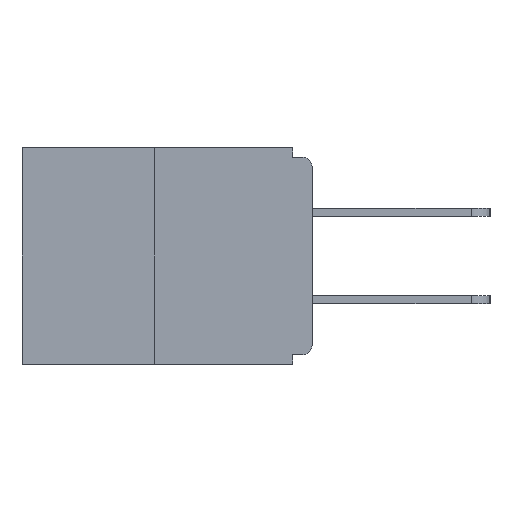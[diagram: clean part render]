
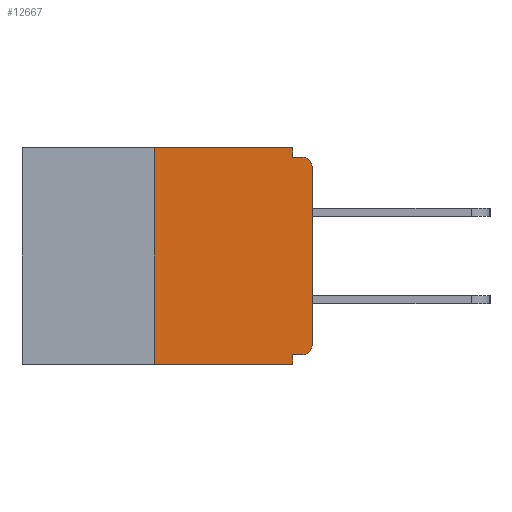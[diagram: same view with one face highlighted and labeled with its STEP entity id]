
A CAD part, left-side view. The second image highlights one B-rep face of the part: STEP entity #12667.
In plain terms, the highlighted planar face has unit normal (-1, 0, 0).
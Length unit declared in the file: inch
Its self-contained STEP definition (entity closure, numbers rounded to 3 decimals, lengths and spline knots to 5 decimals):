
#383 = CARTESIAN_POINT ( 'NONE',  ( 0., 0.25, 0. ) ) ;
#677 = CARTESIAN_POINT ( 'NONE',  ( 0., 0.015, -0.328 ) ) ;
#772 = VERTEX_POINT ( 'NONE', #23433 ) ;
#1003 = LINE ( 'NONE', #21368, #7457 ) ;
#1056 = VECTOR ( 'NONE', #14435, 39.37008 ) ;
#1057 = ORIENTED_EDGE ( 'NONE', *, *, #9455, .F. ) ;
#1495 = CARTESIAN_POINT ( 'NONE',  ( 0., 0., -0.03 ) ) ;
#1531 = DIRECTION ( 'NONE',  ( 0., 0., -1. ) ) ;
#1611 = FACE_OUTER_BOUND ( 'NONE', #10040, .T. ) ;
#2219 = EDGE_CURVE ( 'NONE', #25067, #6807, #1003, .T. ) ;
#2502 = CARTESIAN_POINT ( 'NONE',  ( 0., 0.031, 0. ) ) ;
#2650 = AXIS2_PLACEMENT_3D ( 'NONE', #13484, #15446, #21336 ) ;
#2707 = VERTEX_POINT ( 'NONE', #383 ) ;
#2754 = LINE ( 'NONE', #25011, #20819 ) ;
#3315 = VECTOR ( 'NONE', #22882, 39.37008 ) ;
#3384 = VECTOR ( 'NONE', #14317, 39.37008 ) ;
#3428 = DIRECTION ( 'NONE',  ( 0., 0., 1. ) ) ;
#3651 = ORIENTED_EDGE ( 'NONE', *, *, #4629, .T. ) ;
#3941 = CARTESIAN_POINT ( 'NONE',  ( 0., 0., -0.313 ) ) ;
#4145 = DIRECTION ( 'NONE',  ( 1., 0., 0. ) ) ;
#4515 = EDGE_CURVE ( 'NONE', #20510, #12137, #5167, .T. ) ;
#4629 = EDGE_CURVE ( 'NONE', #15922, #23898, #8237, .T. ) ;
#4657 = EDGE_CURVE ( 'NONE', #17514, #12137, #18951, .T. ) ;
#4662 = CARTESIAN_POINT ( 'NONE',  ( 0., 0.015, -0.03 ) ) ;
#5167 = LINE ( 'NONE', #20684, #3315 ) ;
#5619 = EDGE_CURVE ( 'NONE', #15922, #25067, #13058, .T. ) ;
#6807 = VERTEX_POINT ( 'NONE', #19001 ) ;
#6842 = CARTESIAN_POINT ( 'NONE',  ( 0., 0., -0.328 ) ) ;
#7069 = AXIS2_PLACEMENT_3D ( 'NONE', #10222, #4145, #17853 ) ;
#7457 = VECTOR ( 'NONE', #1531, 39.37008 ) ;
#8237 = CIRCLE ( 'NONE', #2650, 0.015 ) ;
#9455 = EDGE_CURVE ( 'NONE', #772, #20510, #21450, .T. ) ;
#9795 = DIRECTION ( 'NONE',  ( 0., 1., 0. ) ) ;
#10040 = EDGE_LOOP ( 'NONE', ( #16738, #14431, #21371, #14709, #17684, #3651, #24387, #19300, #11890, #1057 ) ) ;
#10222 = CARTESIAN_POINT ( 'NONE',  ( 0., 0.46, 0. ) ) ;
#11515 = LINE ( 'NONE', #12172, #22531 ) ;
#11890 = ORIENTED_EDGE ( 'NONE', *, *, #4515, .F. ) ;
#12075 = VECTOR ( 'NONE', #3428, 39.37008 ) ;
#12137 = VERTEX_POINT ( 'NONE', #16749 ) ;
#12172 = CARTESIAN_POINT ( 'NONE',  ( 0., 0.46, 0. ) ) ;
#12667 = ADVANCED_FACE ( 'NONE', ( #1611 ), #20071, .F. ) ;
#13058 = LINE ( 'NONE', #6842, #15511 ) ;
#13484 = CARTESIAN_POINT ( 'NONE',  ( 0., 0.015, -0.313 ) ) ;
#14317 = DIRECTION ( 'NONE',  ( 0., 0., -1. ) ) ;
#14431 = ORIENTED_EDGE ( 'NONE', *, *, #17342, .F. ) ;
#14435 = DIRECTION ( 'NONE',  ( 0., 0., 1. ) ) ;
#14493 = EDGE_CURVE ( 'NONE', #19205, #6807, #2754, .T. ) ;
#14709 = ORIENTED_EDGE ( 'NONE', *, *, #2219, .F. ) ;
#15285 = DIRECTION ( 'NONE',  ( 0., -1., 0. ) ) ;
#15446 = DIRECTION ( 'NONE',  ( -1., 0., 0. ) ) ;
#15508 = CARTESIAN_POINT ( 'NONE',  ( 0., 0.031, -0.328 ) ) ;
#15511 = VECTOR ( 'NONE', #9795, 39.37008 ) ;
#15762 = LINE ( 'NONE', #17384, #12075 ) ;
#15922 = VERTEX_POINT ( 'NONE', #677 ) ;
#16738 = ORIENTED_EDGE ( 'NONE', *, *, #23455, .F. ) ;
#16749 = CARTESIAN_POINT ( 'NONE',  ( 0., 0.015, -0.015 ) ) ;
#17342 = EDGE_CURVE ( 'NONE', #19205, #2707, #21873, .T. ) ;
#17384 = CARTESIAN_POINT ( 'NONE',  ( 0., 0., 0. ) ) ;
#17514 = VERTEX_POINT ( 'NONE', #1495 ) ;
#17684 = ORIENTED_EDGE ( 'NONE', *, *, #5619, .F. ) ;
#17853 = DIRECTION ( 'NONE',  ( 0., 0., -1. ) ) ;
#18038 = CARTESIAN_POINT ( 'NONE',  ( 0., 0.25, 0. ) ) ;
#18141 = EDGE_CURVE ( 'NONE', #23898, #17514, #15762, .T. ) ;
#18490 = CARTESIAN_POINT ( 'NONE',  ( 0., 0.031, -0.015 ) ) ;
#18872 = CARTESIAN_POINT ( 'NONE',  ( 0., 0.25, -0.343 ) ) ;
#18951 = CIRCLE ( 'NONE', #23277, 0.015 ) ;
#19001 = CARTESIAN_POINT ( 'NONE',  ( 0., 0.031, -0.343 ) ) ;
#19205 = VERTEX_POINT ( 'NONE', #18872 ) ;
#19300 = ORIENTED_EDGE ( 'NONE', *, *, #4657, .T. ) ;
#20071 = PLANE ( 'NONE',  #7069 ) ;
#20096 = DIRECTION ( 'NONE',  ( -1., 0., 0. ) ) ;
#20182 = DIRECTION ( 'NONE',  ( 0., 0., -1. ) ) ;
#20510 = VERTEX_POINT ( 'NONE', #18490 ) ;
#20684 = CARTESIAN_POINT ( 'NONE',  ( 0., 0., -0.015 ) ) ;
#20819 = VECTOR ( 'NONE', #15285, 39.37008 ) ;
#21336 = DIRECTION ( 'NONE',  ( 0., 0., -1. ) ) ;
#21368 = CARTESIAN_POINT ( 'NONE',  ( 0., 0.031, -0.343 ) ) ;
#21371 = ORIENTED_EDGE ( 'NONE', *, *, #14493, .T. ) ;
#21450 = LINE ( 'NONE', #2502, #3384 ) ;
#21672 = DIRECTION ( 'NONE',  ( 0., -1., 0. ) ) ;
#21873 = LINE ( 'NONE', #18038, #1056 ) ;
#22531 = VECTOR ( 'NONE', #21672, 39.37008 ) ;
#22882 = DIRECTION ( 'NONE',  ( 0., -1., 0. ) ) ;
#23277 = AXIS2_PLACEMENT_3D ( 'NONE', #4662, #20096, #20182 ) ;
#23433 = CARTESIAN_POINT ( 'NONE',  ( 0., 0.031, 0. ) ) ;
#23455 = EDGE_CURVE ( 'NONE', #2707, #772, #11515, .T. ) ;
#23898 = VERTEX_POINT ( 'NONE', #3941 ) ;
#24387 = ORIENTED_EDGE ( 'NONE', *, *, #18141, .T. ) ;
#25011 = CARTESIAN_POINT ( 'NONE',  ( 0., 0.46, -0.343 ) ) ;
#25067 = VERTEX_POINT ( 'NONE', #15508 ) ;
